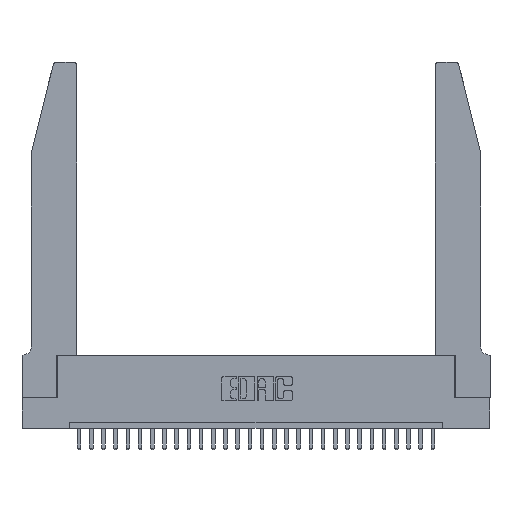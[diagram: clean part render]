
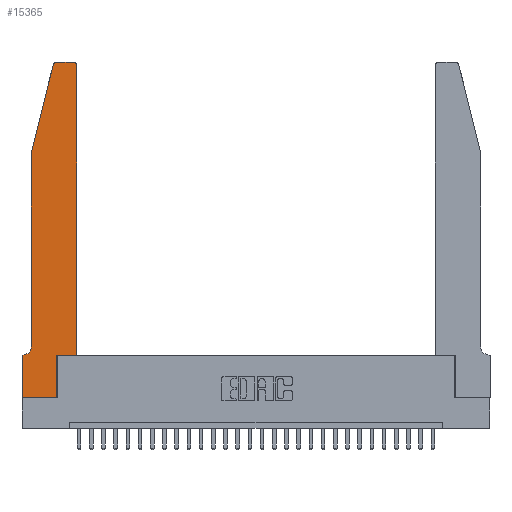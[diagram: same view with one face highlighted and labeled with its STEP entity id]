
A CAD part, top view. The second image highlights one B-rep face of the part: STEP entity #15365.
In plain terms, the highlighted planar face has unit normal (0, 0, 1).
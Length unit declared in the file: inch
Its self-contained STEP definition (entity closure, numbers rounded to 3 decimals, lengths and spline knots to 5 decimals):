
#14 = LINE ( 'NONE', #1560, #23170 ) ;
#112 = CARTESIAN_POINT ( 'NONE',  ( 0., 0., 0.37 ) ) ;
#425 = DIRECTION ( 'NONE',  ( 0., -1., 0. ) ) ;
#569 = VERTEX_POINT ( 'NONE', #20851 ) ;
#772 = DIRECTION ( 'NONE',  ( 0., 1., 0. ) ) ;
#1073 = VERTEX_POINT ( 'NONE', #6607 ) ;
#1118 = ORIENTED_EDGE ( 'NONE', *, *, #9600, .T. ) ;
#1390 = CIRCLE ( 'NONE', #6703, 0.03 ) ;
#1501 = EDGE_CURVE ( 'NONE', #12982, #569, #5733, .T. ) ;
#1560 = CARTESIAN_POINT ( 'NONE',  ( 0.4505, 0.35, 0.37 ) ) ;
#1902 = VECTOR ( 'NONE', #8102, 39.37008 ) ;
#2206 = VECTOR ( 'NONE', #7571, 39.37008 ) ;
#2698 = EDGE_CURVE ( 'NONE', #26158, #26576, #14394, .T. ) ;
#3356 = DIRECTION ( 'NONE',  ( 1., 0., 0. ) ) ;
#3808 = CARTESIAN_POINT ( 'NONE',  ( 0.0755, 2., 0.37 ) ) ;
#4945 = VECTOR ( 'NONE', #15181, 39.37008 ) ;
#4987 = VECTOR ( 'NONE', #15597, 39.37008 ) ;
#5072 = ORIENTED_EDGE ( 'NONE', *, *, #10514, .T. ) ;
#5729 = LINE ( 'NONE', #27382, #1902 ) ;
#5733 = CIRCLE ( 'NONE', #25280, 0.03 ) ;
#6034 = DIRECTION ( 'NONE',  ( 1., 0., 0. ) ) ;
#6067 = DIRECTION ( 'NONE',  ( -0.239, -0.971, 0. ) ) ;
#6258 = DIRECTION ( 'NONE',  ( 1., 0., 0. ) ) ;
#6607 = CARTESIAN_POINT ( 'NONE',  ( 0.2865, 0., 0.37 ) ) ;
#6703 = AXIS2_PLACEMENT_3D ( 'NONE', #20937, #14197, #21030 ) ;
#7378 = EDGE_CURVE ( 'NONE', #20454, #26557, #1390, .T. ) ;
#7437 = LINE ( 'NONE', #20825, #27139 ) ;
#7571 = DIRECTION ( 'NONE',  ( -1., 0., 0. ) ) ;
#8102 = DIRECTION ( 'NONE',  ( -1., 0., 0. ) ) ;
#8607 = ORIENTED_EDGE ( 'NONE', *, *, #12224, .T. ) ;
#9005 = CARTESIAN_POINT ( 'NONE',  ( 0.0055, 0.35, 0.37 ) ) ;
#9265 = CIRCLE ( 'NONE', #24354, 0.07 ) ;
#9600 = EDGE_CURVE ( 'NONE', #1073, #25855, #19852, .T. ) ;
#9734 = CARTESIAN_POINT ( 'NONE',  ( 0.0755, 0.35, 0.37 ) ) ;
#10241 = EDGE_CURVE ( 'NONE', #26557, #12982, #5729, .T. ) ;
#10414 = ORIENTED_EDGE ( 'NONE', *, *, #1501, .T. ) ;
#10429 = ORIENTED_EDGE ( 'NONE', *, *, #22316, .T. ) ;
#10514 = EDGE_CURVE ( 'NONE', #17103, #19246, #7437, .T. ) ;
#10638 = CARTESIAN_POINT ( 'NONE',  ( 0.284, 2.72, 0.37 ) ) ;
#11373 = EDGE_CURVE ( 'NONE', #27008, #20454, #23951, .T. ) ;
#12224 = EDGE_CURVE ( 'NONE', #26576, #27529, #9265, .T. ) ;
#12597 = CARTESIAN_POINT ( 'NONE',  ( 0., 0.35, 0.37 ) ) ;
#12982 = VERTEX_POINT ( 'NONE', #26862 ) ;
#13724 = EDGE_CURVE ( 'NONE', #27529, #17103, #15130, .T. ) ;
#13791 = VECTOR ( 'NONE', #772, 39.37008 ) ;
#14197 = DIRECTION ( 'NONE',  ( 0., 0., 1. ) ) ;
#14394 = LINE ( 'NONE', #20048, #4987 ) ;
#14975 = CARTESIAN_POINT ( 'NONE',  ( 0.4505, 0.35, 0.37 ) ) ;
#15130 = LINE ( 'NONE', #9734, #2206 ) ;
#15181 = DIRECTION ( 'NONE',  ( 0., 1., 0. ) ) ;
#15365 = ADVANCED_FACE ( 'NONE', ( #27699 ), #26140, .T. ) ;
#15562 = ORIENTED_EDGE ( 'NONE', *, *, #25488, .T. ) ;
#15571 = VECTOR ( 'NONE', #6067, 39.37008 ) ;
#15597 = DIRECTION ( 'NONE',  ( 0., -1., 0. ) ) ;
#16713 = CARTESIAN_POINT ( 'NONE',  ( 0.0755, 0.42, 0.37 ) ) ;
#16800 = CARTESIAN_POINT ( 'NONE',  ( 0., 0.35, 0.37 ) ) ;
#17103 = VERTEX_POINT ( 'NONE', #16800 ) ;
#17360 = ORIENTED_EDGE ( 'NONE', *, *, #2698, .T. ) ;
#17672 = ORIENTED_EDGE ( 'NONE', *, *, #7378, .T. ) ;
#17813 = DIRECTION ( 'NONE',  ( 0., 0., 1. ) ) ;
#19065 = DIRECTION ( 'NONE',  ( 0., 0., -1. ) ) ;
#19246 = VERTEX_POINT ( 'NONE', #112 ) ;
#19852 = LINE ( 'NONE', #20784, #13791 ) ;
#20048 = CARTESIAN_POINT ( 'NONE',  ( 0.0755, 2., 0.37 ) ) ;
#20454 = VERTEX_POINT ( 'NONE', #21375 ) ;
#20784 = CARTESIAN_POINT ( 'NONE',  ( 0.2865, 0.35, 0.37 ) ) ;
#20825 = CARTESIAN_POINT ( 'NONE',  ( 0., 0., 0.37 ) ) ;
#20851 = CARTESIAN_POINT ( 'NONE',  ( 0.25487, 2.72718, 0.37 ) ) ;
#20937 = CARTESIAN_POINT ( 'NONE',  ( 0.4205, 2.72, 0.37 ) ) ;
#21030 = DIRECTION ( 'NONE',  ( 1., 0., 0. ) ) ;
#21227 = ORIENTED_EDGE ( 'NONE', *, *, #13724, .T. ) ;
#21375 = CARTESIAN_POINT ( 'NONE',  ( 0.4505, 2.72, 0.37 ) ) ;
#21884 = CARTESIAN_POINT ( 'NONE',  ( 0.0755, 2., 0.37 ) ) ;
#22316 = EDGE_CURVE ( 'NONE', #569, #26158, #23011, .T. ) ;
#22698 = CARTESIAN_POINT ( 'NONE',  ( 0.4505, 0.35, 0.37 ) ) ;
#22821 = ORIENTED_EDGE ( 'NONE', *, *, #26780, .T. ) ;
#22849 = CARTESIAN_POINT ( 'NONE',  ( 0.2865, 0.35, 0.37 ) ) ;
#23011 = LINE ( 'NONE', #21884, #15571 ) ;
#23170 = VECTOR ( 'NONE', #6034, 39.37008 ) ;
#23332 = VECTOR ( 'NONE', #3356, 39.37008 ) ;
#23874 = CARTESIAN_POINT ( 'NONE',  ( 0., 0., 0.37 ) ) ;
#23877 = ORIENTED_EDGE ( 'NONE', *, *, #10241, .T. ) ;
#23951 = LINE ( 'NONE', #14975, #4945 ) ;
#24094 = DIRECTION ( 'NONE',  ( 1., 0., 0. ) ) ;
#24354 = AXIS2_PLACEMENT_3D ( 'NONE', #27896, #19065, #28099 ) ;
#25121 = CARTESIAN_POINT ( 'NONE',  ( 0.4205, 2.75, 0.37 ) ) ;
#25280 = AXIS2_PLACEMENT_3D ( 'NONE', #10638, #17813, #6258 ) ;
#25488 = EDGE_CURVE ( 'NONE', #19246, #1073, #26547, .T. ) ;
#25855 = VERTEX_POINT ( 'NONE', #22849 ) ;
#25864 = AXIS2_PLACEMENT_3D ( 'NONE', #12597, #28586, #24094 ) ;
#26140 = PLANE ( 'NONE',  #25864 ) ;
#26158 = VERTEX_POINT ( 'NONE', #3808 ) ;
#26547 = LINE ( 'NONE', #23874, #23332 ) ;
#26557 = VERTEX_POINT ( 'NONE', #25121 ) ;
#26576 = VERTEX_POINT ( 'NONE', #16713 ) ;
#26780 = EDGE_CURVE ( 'NONE', #25855, #27008, #14, .T. ) ;
#26862 = CARTESIAN_POINT ( 'NONE',  ( 0.284, 2.75, 0.37 ) ) ;
#27008 = VERTEX_POINT ( 'NONE', #22698 ) ;
#27139 = VECTOR ( 'NONE', #425, 39.37008 ) ;
#27382 = CARTESIAN_POINT ( 'NONE',  ( 0.2605, 2.75, 0.37 ) ) ;
#27529 = VERTEX_POINT ( 'NONE', #9005 ) ;
#27699 = FACE_OUTER_BOUND ( 'NONE', #27743, .T. ) ;
#27743 = EDGE_LOOP ( 'NONE', ( #23877, #10414, #10429, #17360, #8607, #21227, #5072, #15562, #1118, #22821, #28082, #17672 ) ) ;
#27896 = CARTESIAN_POINT ( 'NONE',  ( 0.0055, 0.42, 0.37 ) ) ;
#28082 = ORIENTED_EDGE ( 'NONE', *, *, #11373, .T. ) ;
#28099 = DIRECTION ( 'NONE',  ( -1., 0., 0. ) ) ;
#28586 = DIRECTION ( 'NONE',  ( 0., 0., 1. ) ) ;
